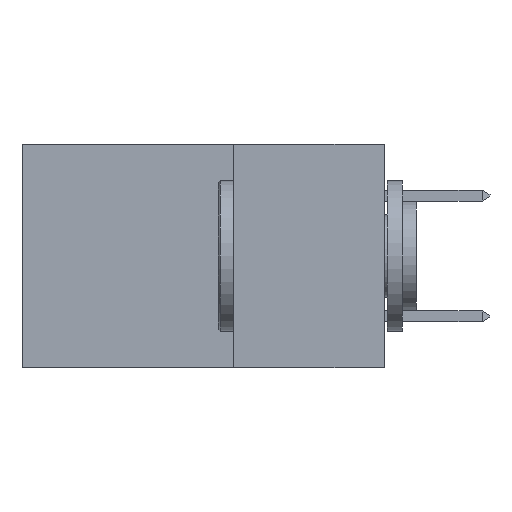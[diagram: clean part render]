
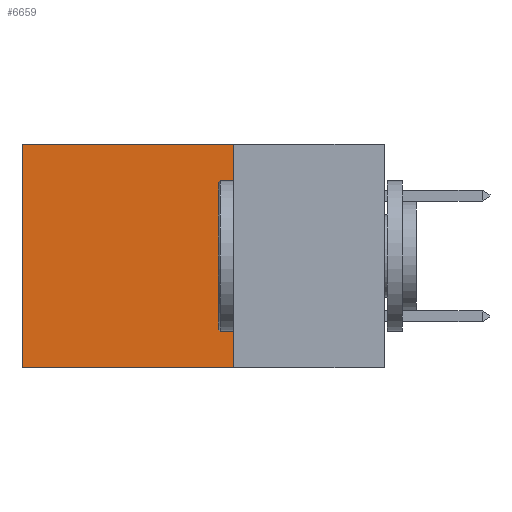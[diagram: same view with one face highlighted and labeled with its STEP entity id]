
A CAD part, left-side view. The second image highlights one B-rep face of the part: STEP entity #6659.
In plain terms, the highlighted planar face has unit normal (-1, 0, 0).
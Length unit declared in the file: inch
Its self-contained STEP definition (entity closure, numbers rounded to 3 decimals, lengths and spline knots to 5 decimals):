
#34 = DIRECTION ( 'NONE',  ( 0., 1., 0. ) ) ;
#132 = EDGE_CURVE ( 'NONE', #20638, #7141, #7097, .T. ) ;
#565 = AXIS2_PLACEMENT_3D ( 'NONE', #17728, #21143, #10852 ) ;
#1924 = VERTEX_POINT ( 'NONE', #4243 ) ;
#3437 = ORIENTED_EDGE ( 'NONE', *, *, #132, .F. ) ;
#4243 = CARTESIAN_POINT ( 'NONE',  ( 0.2875, 0.6, 0. ) ) ;
#4315 = VECTOR ( 'NONE', #21432, 39.37008 ) ;
#4484 = EDGE_CURVE ( 'NONE', #18819, #20638, #4854, .T. ) ;
#4854 = LINE ( 'NONE', #21067, #4315 ) ;
#4958 = LINE ( 'NONE', #17880, #13473 ) ;
#6578 = VECTOR ( 'NONE', #15506, 39.37008 ) ;
#6659 = ADVANCED_FACE ( 'NONE', ( #21779 ), #12542, .F. ) ;
#6989 = CARTESIAN_POINT ( 'NONE',  ( 0.2875, 0.6, -0.37 ) ) ;
#7097 = LINE ( 'NONE', #15529, #6578 ) ;
#7141 = VERTEX_POINT ( 'NONE', #6989 ) ;
#8075 = EDGE_CURVE ( 'NONE', #1924, #7141, #4958, .T. ) ;
#8486 = EDGE_LOOP ( 'NONE', ( #17188, #3437, #16056, #9980 ) ) ;
#9980 = ORIENTED_EDGE ( 'NONE', *, *, #12401, .T. ) ;
#10248 = CARTESIAN_POINT ( 'NONE',  ( 0.2875, 0.25, 0. ) ) ;
#10852 = DIRECTION ( 'NONE',  ( 0., 0., -1. ) ) ;
#12232 = VECTOR ( 'NONE', #34, 39.37008 ) ;
#12401 = EDGE_CURVE ( 'NONE', #18819, #1924, #17348, .T. ) ;
#12542 = PLANE ( 'NONE',  #565 ) ;
#13113 = CARTESIAN_POINT ( 'NONE',  ( 0.2875, 0.25, 0. ) ) ;
#13473 = VECTOR ( 'NONE', #19590, 39.37008 ) ;
#15506 = DIRECTION ( 'NONE',  ( 0., 1., 0. ) ) ;
#15529 = CARTESIAN_POINT ( 'NONE',  ( 0.2875, 0.25, -0.37 ) ) ;
#16056 = ORIENTED_EDGE ( 'NONE', *, *, #4484, .F. ) ;
#17188 = ORIENTED_EDGE ( 'NONE', *, *, #8075, .T. ) ;
#17348 = LINE ( 'NONE', #10248, #12232 ) ;
#17728 = CARTESIAN_POINT ( 'NONE',  ( 0.2875, 0.25, 0. ) ) ;
#17880 = CARTESIAN_POINT ( 'NONE',  ( 0.2875, 0.6, 0. ) ) ;
#18819 = VERTEX_POINT ( 'NONE', #13113 ) ;
#19590 = DIRECTION ( 'NONE',  ( 0., 0., -1. ) ) ;
#20638 = VERTEX_POINT ( 'NONE', #21482 ) ;
#21067 = CARTESIAN_POINT ( 'NONE',  ( 0.2875, 0.25, 0. ) ) ;
#21143 = DIRECTION ( 'NONE',  ( 1., 0., 0. ) ) ;
#21432 = DIRECTION ( 'NONE',  ( 0., 0., -1. ) ) ;
#21482 = CARTESIAN_POINT ( 'NONE',  ( 0.2875, 0.25, -0.37 ) ) ;
#21779 = FACE_OUTER_BOUND ( 'NONE', #8486, .T. ) ;
